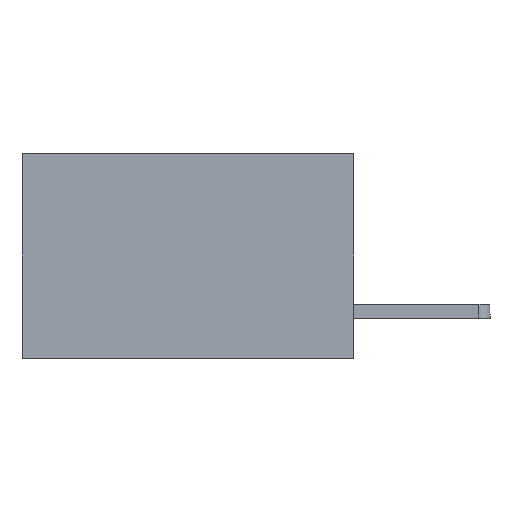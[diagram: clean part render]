
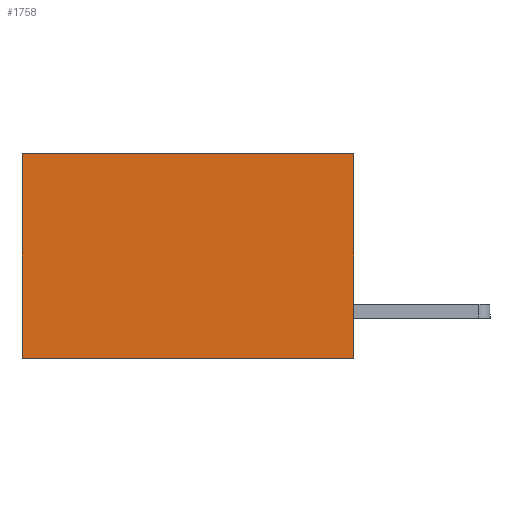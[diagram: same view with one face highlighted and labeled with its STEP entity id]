
A CAD part, left-side view. The second image highlights one B-rep face of the part: STEP entity #1758.
In plain terms, the highlighted planar face has unit normal (-1, 0, 0).
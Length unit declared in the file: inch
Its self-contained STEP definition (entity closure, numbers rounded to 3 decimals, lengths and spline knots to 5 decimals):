
#517 = DIRECTION ( 'NONE',  ( 1., 0., 0. ) ) ;
#569 = VECTOR ( 'NONE', #711, 39.37008 ) ;
#625 = VERTEX_POINT ( 'NONE', #3131 ) ;
#711 = DIRECTION ( 'NONE',  ( 0., 0., -1. ) ) ;
#729 = EDGE_LOOP ( 'NONE', ( #4761, #4748, #8221, #8242 ) ) ;
#1476 = VERTEX_POINT ( 'NONE', #5371 ) ;
#1758 = ADVANCED_FACE ( 'NONE', ( #7104 ), #2202, .F. ) ;
#1840 = EDGE_CURVE ( 'NONE', #1476, #625, #8205, .T. ) ;
#1995 = VECTOR ( 'NONE', #6404, 39.37008 ) ;
#2202 = PLANE ( 'NONE',  #6614 ) ;
#2261 = CARTESIAN_POINT ( 'NONE',  ( 0.2875, 0., 0. ) ) ;
#2501 = VERTEX_POINT ( 'NONE', #8116 ) ;
#2524 = DIRECTION ( 'NONE',  ( 0., 1., 0. ) ) ;
#3131 = CARTESIAN_POINT ( 'NONE',  ( 0.2875, 0.6, -0.37 ) ) ;
#3194 = LINE ( 'NONE', #6128, #569 ) ;
#3706 = CARTESIAN_POINT ( 'NONE',  ( 0.2875, 0., 0. ) ) ;
#3737 = CARTESIAN_POINT ( 'NONE',  ( 0.2875, 0., -0.37 ) ) ;
#3793 = CARTESIAN_POINT ( 'NONE',  ( 0.2875, 0., 0. ) ) ;
#4748 = ORIENTED_EDGE ( 'NONE', *, *, #1840, .F. ) ;
#4761 = ORIENTED_EDGE ( 'NONE', *, *, #5198, .T. ) ;
#4778 = EDGE_CURVE ( 'NONE', #6420, #2501, #6793, .T. ) ;
#4848 = CARTESIAN_POINT ( 'NONE',  ( 0.2875, 0., 0. ) ) ;
#4880 = VECTOR ( 'NONE', #8439, 39.37008 ) ;
#5198 = EDGE_CURVE ( 'NONE', #2501, #625, #3194, .T. ) ;
#5371 = CARTESIAN_POINT ( 'NONE',  ( 0.2875, 0., -0.37 ) ) ;
#6128 = CARTESIAN_POINT ( 'NONE',  ( 0.2875, 0.6, 0. ) ) ;
#6404 = DIRECTION ( 'NONE',  ( 0., 0., -1. ) ) ;
#6420 = VERTEX_POINT ( 'NONE', #4848 ) ;
#6490 = VECTOR ( 'NONE', #2524, 39.37008 ) ;
#6614 = AXIS2_PLACEMENT_3D ( 'NONE', #3706, #517, #7229 ) ;
#6793 = LINE ( 'NONE', #3793, #4880 ) ;
#7104 = FACE_OUTER_BOUND ( 'NONE', #729, .T. ) ;
#7229 = DIRECTION ( 'NONE',  ( 0., 0., -1. ) ) ;
#7496 = EDGE_CURVE ( 'NONE', #6420, #1476, #7521, .T. ) ;
#7521 = LINE ( 'NONE', #2261, #1995 ) ;
#8116 = CARTESIAN_POINT ( 'NONE',  ( 0.2875, 0.6, 0. ) ) ;
#8205 = LINE ( 'NONE', #3737, #6490 ) ;
#8221 = ORIENTED_EDGE ( 'NONE', *, *, #7496, .F. ) ;
#8242 = ORIENTED_EDGE ( 'NONE', *, *, #4778, .T. ) ;
#8439 = DIRECTION ( 'NONE',  ( 0., 1., 0. ) ) ;
